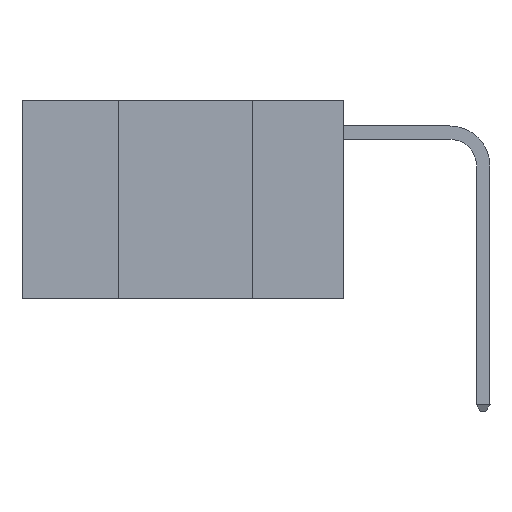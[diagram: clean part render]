
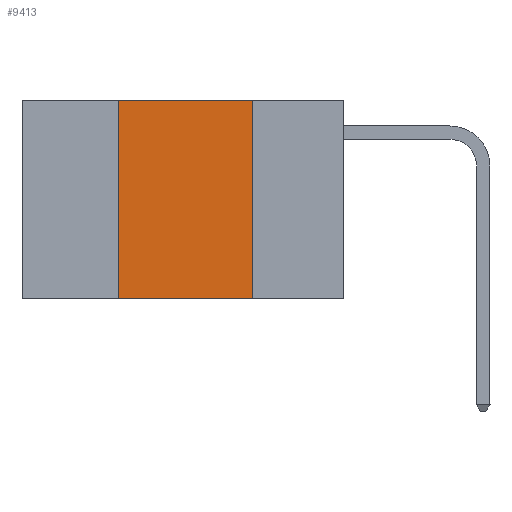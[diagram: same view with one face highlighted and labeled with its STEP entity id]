
A CAD part, left-side view. The second image highlights one B-rep face of the part: STEP entity #9413.
In plain terms, the highlighted planar face has unit normal (-1, 0, 0).
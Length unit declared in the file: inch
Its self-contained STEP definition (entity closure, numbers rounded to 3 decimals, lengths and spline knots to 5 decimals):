
#91 = CARTESIAN_POINT ( 'NONE',  ( 0., 0.42, 0. ) ) ;
#690 = CARTESIAN_POINT ( 'NONE',  ( 0., 0.42, 0. ) ) ;
#783 = EDGE_CURVE ( 'NONE', #7610, #1299, #8919, .T. ) ;
#1116 = EDGE_CURVE ( 'NONE', #14178, #7610, #10681, .T. ) ;
#1228 = CARTESIAN_POINT ( 'NONE',  ( 0., 0.17, 0. ) ) ;
#1299 = VERTEX_POINT ( 'NONE', #1725 ) ;
#1725 = CARTESIAN_POINT ( 'NONE',  ( 0., 0.17, -0.37 ) ) ;
#2033 = DIRECTION ( 'NONE',  ( 0., -1., 0. ) ) ;
#2935 = AXIS2_PLACEMENT_3D ( 'NONE', #3318, #12455, #4506 ) ;
#2997 = LINE ( 'NONE', #13555, #7269 ) ;
#3316 = EDGE_CURVE ( 'NONE', #14420, #14178, #10945, .T. ) ;
#3318 = CARTESIAN_POINT ( 'NONE',  ( 0., 0.6, 0. ) ) ;
#4506 = DIRECTION ( 'NONE',  ( 0., 0., -1. ) ) ;
#5135 = VECTOR ( 'NONE', #8685, 39.37008 ) ;
#5263 = DIRECTION ( 'NONE',  ( 0., 0., 1. ) ) ;
#5615 = FACE_OUTER_BOUND ( 'NONE', #13370, .T. ) ;
#5852 = ORIENTED_EDGE ( 'NONE', *, *, #1116, .F. ) ;
#6302 = ORIENTED_EDGE ( 'NONE', *, *, #3316, .F. ) ;
#7076 = DIRECTION ( 'NONE',  ( 0., -1., 0. ) ) ;
#7269 = VECTOR ( 'NONE', #2033, 39.37008 ) ;
#7610 = VERTEX_POINT ( 'NONE', #1228 ) ;
#8544 = ORIENTED_EDGE ( 'NONE', *, *, #10857, .T. ) ;
#8685 = DIRECTION ( 'NONE',  ( 0., 0., -1. ) ) ;
#8833 = VECTOR ( 'NONE', #5263, 39.37008 ) ;
#8919 = LINE ( 'NONE', #12473, #5135 ) ;
#9331 = ORIENTED_EDGE ( 'NONE', *, *, #783, .F. ) ;
#9413 = ADVANCED_FACE ( 'NONE', ( #5615 ), #13628, .F. ) ;
#10681 = LINE ( 'NONE', #12894, #14740 ) ;
#10857 = EDGE_CURVE ( 'NONE', #14420, #1299, #2997, .T. ) ;
#10945 = LINE ( 'NONE', #690, #8833 ) ;
#12455 = DIRECTION ( 'NONE',  ( 1., 0., 0. ) ) ;
#12473 = CARTESIAN_POINT ( 'NONE',  ( 0., 0.17, 0. ) ) ;
#12894 = CARTESIAN_POINT ( 'NONE',  ( 0., 0.6, 0. ) ) ;
#13370 = EDGE_LOOP ( 'NONE', ( #9331, #5852, #6302, #8544 ) ) ;
#13555 = CARTESIAN_POINT ( 'NONE',  ( 0., 0.6, -0.37 ) ) ;
#13622 = CARTESIAN_POINT ( 'NONE',  ( 0., 0.42, -0.37 ) ) ;
#13628 = PLANE ( 'NONE',  #2935 ) ;
#14178 = VERTEX_POINT ( 'NONE', #91 ) ;
#14420 = VERTEX_POINT ( 'NONE', #13622 ) ;
#14740 = VECTOR ( 'NONE', #7076, 39.37008 ) ;
